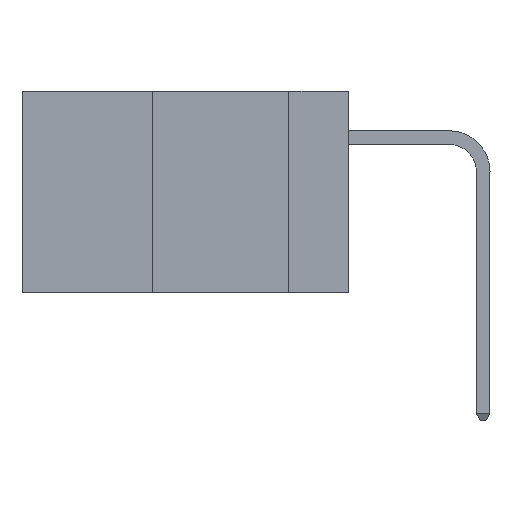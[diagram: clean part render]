
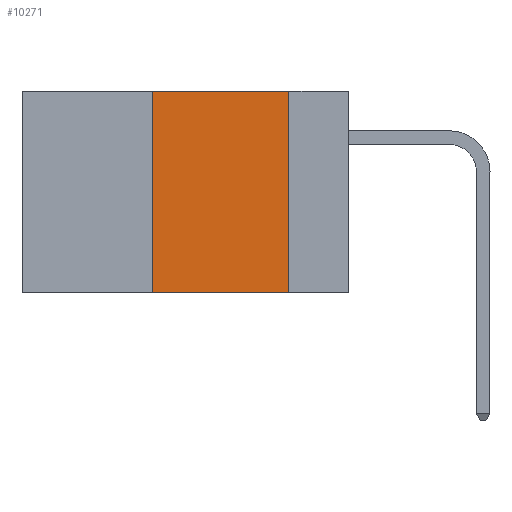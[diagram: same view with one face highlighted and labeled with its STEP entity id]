
A CAD part, left-side view. The second image highlights one B-rep face of the part: STEP entity #10271.
In plain terms, the highlighted planar face has unit normal (-1, 0, 0).
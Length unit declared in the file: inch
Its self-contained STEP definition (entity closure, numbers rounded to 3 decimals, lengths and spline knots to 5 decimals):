
#113 = FACE_OUTER_BOUND ( 'NONE', #10994, .T. ) ;
#1536 = ORIENTED_EDGE ( 'NONE', *, *, #6825, .F. ) ;
#1767 = LINE ( 'NONE', #18777, #10127 ) ;
#6560 = EDGE_CURVE ( 'NONE', #17775, #12777, #6881, .T. ) ;
#6561 = AXIS2_PLACEMENT_3D ( 'NONE', #13844, #29653, #9385 ) ;
#6825 = EDGE_CURVE ( 'NONE', #17775, #12795, #1767, .T. ) ;
#6881 = LINE ( 'NONE', #24718, #25260 ) ;
#7481 = CARTESIAN_POINT ( 'NONE',  ( 0., 0.36, 0. ) ) ;
#8540 = DIRECTION ( 'NONE',  ( 0., -1., 0. ) ) ;
#9311 = LINE ( 'NONE', #15588, #20821 ) ;
#9385 = DIRECTION ( 'NONE',  ( 0., 0., -1. ) ) ;
#10127 = VECTOR ( 'NONE', #20965, 39.37008 ) ;
#10271 = ADVANCED_FACE ( 'NONE', ( #113 ), #11214, .F. ) ;
#10994 = EDGE_LOOP ( 'NONE', ( #19923, #15995, #1536, #19121 ) ) ;
#11140 = CARTESIAN_POINT ( 'NONE',  ( 0., 0.6, 0. ) ) ;
#11214 = PLANE ( 'NONE',  #6561 ) ;
#11251 = VECTOR ( 'NONE', #8540, 39.37008 ) ;
#12777 = VERTEX_POINT ( 'NONE', #18877 ) ;
#12795 = VERTEX_POINT ( 'NONE', #7481 ) ;
#13256 = DIRECTION ( 'NONE',  ( 0., 0., -1. ) ) ;
#13844 = CARTESIAN_POINT ( 'NONE',  ( 0., 0.6, 0. ) ) ;
#14908 = EDGE_CURVE ( 'NONE', #12795, #20431, #20585, .T. ) ;
#15588 = CARTESIAN_POINT ( 'NONE',  ( 0., 0.11, 0. ) ) ;
#15677 = DIRECTION ( 'NONE',  ( 0., -1., 0. ) ) ;
#15995 = ORIENTED_EDGE ( 'NONE', *, *, #14908, .F. ) ;
#17775 = VERTEX_POINT ( 'NONE', #28724 ) ;
#18777 = CARTESIAN_POINT ( 'NONE',  ( 0., 0.36, 0. ) ) ;
#18877 = CARTESIAN_POINT ( 'NONE',  ( 0., 0.11, -0.37 ) ) ;
#19121 = ORIENTED_EDGE ( 'NONE', *, *, #6560, .T. ) ;
#19923 = ORIENTED_EDGE ( 'NONE', *, *, #27620, .F. ) ;
#20431 = VERTEX_POINT ( 'NONE', #20483 ) ;
#20483 = CARTESIAN_POINT ( 'NONE',  ( 0., 0.11, 0. ) ) ;
#20585 = LINE ( 'NONE', #11140, #11251 ) ;
#20821 = VECTOR ( 'NONE', #13256, 39.37008 ) ;
#20965 = DIRECTION ( 'NONE',  ( 0., 0., 1. ) ) ;
#24718 = CARTESIAN_POINT ( 'NONE',  ( 0., 0.6, -0.37 ) ) ;
#25260 = VECTOR ( 'NONE', #15677, 39.37008 ) ;
#27620 = EDGE_CURVE ( 'NONE', #20431, #12777, #9311, .T. ) ;
#28724 = CARTESIAN_POINT ( 'NONE',  ( 0., 0.36, -0.37 ) ) ;
#29653 = DIRECTION ( 'NONE',  ( 1., 0., 0. ) ) ;
